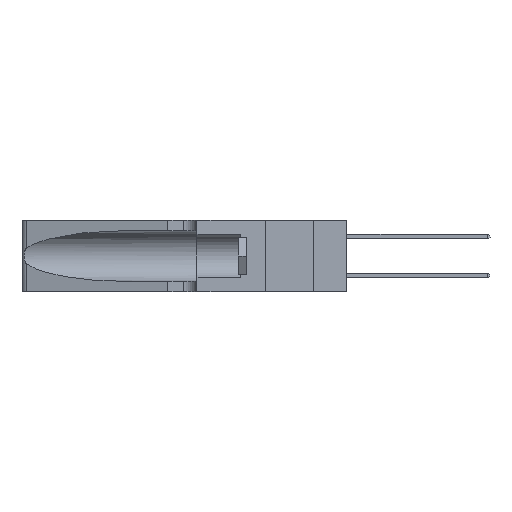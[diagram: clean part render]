
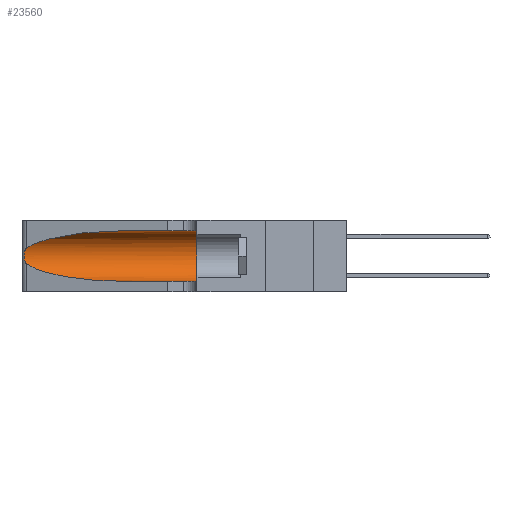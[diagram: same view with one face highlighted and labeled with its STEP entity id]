
A CAD part, left-side view. The second image highlights one B-rep face of the part: STEP entity #23560.
In plain terms, the highlighted cylindrical face has radius 3.308 mm (diameter 6.617 mm), a partial arc.
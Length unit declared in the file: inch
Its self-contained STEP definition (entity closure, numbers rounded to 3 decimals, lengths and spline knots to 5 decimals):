
#1536 = CARTESIAN_POINT ( 'NONE',  ( 0.1305, 0.35, 0.185 ) ) ;
#1537 = ORIENTED_EDGE ( 'NONE', *, *, #2517, .T. ) ;
#1906 = VECTOR ( 'NONE', #22096, 39.37008 ) ;
#1913 =( BOUNDED_CURVE ( )  B_SPLINE_CURVE ( 3, ( #11397, #3986, #19092, #2240 ),
 .UNSPECIFIED., .F., .T. ) 
 B_SPLINE_CURVE_WITH_KNOTS ( ( 4, 4 ),
 ( 1.5708, 2.84003 ),
 .UNSPECIFIED. ) 
 CURVE ( )  GEOMETRIC_REPRESENTATION_ITEM ( )  RATIONAL_B_SPLINE_CURVE ( ( 1., 0.87, 0.87, 1. ) ) 
 REPRESENTATION_ITEM ( '' )  );
#2240 = CARTESIAN_POINT ( 'NONE',  ( 0.25487, 1.22718, 0.22369 ) ) ;
#2402 = CARTESIAN_POINT ( 'NONE',  ( 0.25789, 1.23486, 0.15765 ) ) ;
#2517 = EDGE_CURVE ( 'NONE', #20224, #18466, #10002, .T. ) ;
#2695 = CARTESIAN_POINT ( 'NONE',  ( 0.25487, 1.22718, 0.14631 ) ) ;
#3182 = CARTESIAN_POINT ( 'NONE',  ( 0.25487, 1.22718, 0.14631 ) ) ;
#3450 = DIRECTION ( 'NONE',  ( 0., 1., 0. ) ) ;
#3831 = CIRCLE ( 'NONE', #10021, 0.13025 ) ;
#3986 = CARTESIAN_POINT ( 'NONE',  ( 0.18966, 0.96281, 0.31525 ) ) ;
#4203 = VERTEX_POINT ( 'NONE', #20815 ) ;
#4675 = AXIS2_PLACEMENT_3D ( 'NONE', #20613, #13073, #16848 ) ;
#4845 = VECTOR ( 'NONE', #14578, 39.37008 ) ;
#5646 = B_SPLINE_CURVE_WITH_KNOTS ( 'NONE', 3,
 ( #23398, #12052, #15802, #23474, #6324, #13970, #11973, #15642, #17812, #6080, #2402, #17571, #23313, #7895 ),
 .UNSPECIFIED., .F., .F.,
 ( 4, 2, 2, 2, 2, 2, 4 ),
 ( 0., 0.00027, 0.00053, 0.00107, 0.0016, 0.00187, 0.00214 ),
 .UNSPECIFIED. ) ;
#5675 = EDGE_CURVE ( 'NONE', #18481, #15264, #1913, .T. ) ;
#6080 = CARTESIAN_POINT ( 'NONE',  ( 0.25856, 1.23593, 0.16098 ) ) ;
#6324 = CARTESIAN_POINT ( 'NONE',  ( 0.25854, 1.2359, 0.20912 ) ) ;
#6445 = CARTESIAN_POINT ( 'NONE',  ( 0.1305, 0.35, 0.31525 ) ) ;
#6606 = CARTESIAN_POINT ( 'NONE',  ( 0.1305, 0.72297, 0.05475 ) ) ;
#6783 = CARTESIAN_POINT ( 'NONE',  ( 0.1305, 1.61858, 0.05475 ) ) ;
#6991 = ORIENTED_EDGE ( 'NONE', *, *, #23444, .T. ) ;
#7621 = EDGE_CURVE ( 'NONE', #19948, #4203, #3831, .T. ) ;
#7828 = LINE ( 'NONE', #9065, #4845 ) ;
#7895 = CARTESIAN_POINT ( 'NONE',  ( 0.25487, 1.22718, 0.14631 ) ) ;
#8042 = ORIENTED_EDGE ( 'NONE', *, *, #15702, .T. ) ;
#8195 = CARTESIAN_POINT ( 'NONE',  ( 0.18966, 0.96281, 0.05475 ) ) ;
#9065 = CARTESIAN_POINT ( 'NONE',  ( 0.1305, 1.61858, 0.31525 ) ) ;
#10002 =( BOUNDED_CURVE ( )  B_SPLINE_CURVE ( 3, ( #2695, #21771, #8195, #6606 ),
 .UNSPECIFIED., .F., .F. ) 
 B_SPLINE_CURVE_WITH_KNOTS ( ( 4, 4 ),
 ( 3.44316, 4.71239 ),
 .UNSPECIFIED. ) 
 CURVE ( )  GEOMETRIC_REPRESENTATION_ITEM ( )  RATIONAL_B_SPLINE_CURVE ( ( 1., 0.87, 0.87, 1. ) ) 
 REPRESENTATION_ITEM ( '' )  );
#10021 = AXIS2_PLACEMENT_3D ( 'NONE', #1536, #3450, #16776 ) ;
#11397 = CARTESIAN_POINT ( 'NONE',  ( 0.1305, 0.72297, 0.31525 ) ) ;
#11741 = CARTESIAN_POINT ( 'NONE',  ( 0.1305, 0.72297, 0.31525 ) ) ;
#11766 = ORIENTED_EDGE ( 'NONE', *, *, #24128, .F. ) ;
#11973 = CARTESIAN_POINT ( 'NONE',  ( 0.26075, 1.23896, 0.19203 ) ) ;
#12052 = CARTESIAN_POINT ( 'NONE',  ( 0.25555, 1.22994, 0.2215 ) ) ;
#13073 = DIRECTION ( 'NONE',  ( 0., -1., 0. ) ) ;
#13970 = CARTESIAN_POINT ( 'NONE',  ( 0.26018, 1.23835, 0.19895 ) ) ;
#14418 = CYLINDRICAL_SURFACE ( 'NONE', #4675, 0.13025 ) ;
#14571 = CARTESIAN_POINT ( 'NONE',  ( 0.25487, 1.22718, 0.22369 ) ) ;
#14578 = DIRECTION ( 'NONE',  ( 0., -1., 0. ) ) ;
#15264 = VERTEX_POINT ( 'NONE', #14571 ) ;
#15642 = CARTESIAN_POINT ( 'NONE',  ( 0.26075, 1.23896, 0.178 ) ) ;
#15702 = EDGE_CURVE ( 'NONE', #15264, #20224, #5646, .T. ) ;
#15802 = CARTESIAN_POINT ( 'NONE',  ( 0.25639, 1.23184, 0.21858 ) ) ;
#16776 = DIRECTION ( 'NONE',  ( 0., 0., 1. ) ) ;
#16848 = DIRECTION ( 'NONE',  ( 0., 0., -1. ) ) ;
#17571 = CARTESIAN_POINT ( 'NONE',  ( 0.25639, 1.23186, 0.15144 ) ) ;
#17812 = CARTESIAN_POINT ( 'NONE',  ( 0.26017, 1.23833, 0.17102 ) ) ;
#18466 = VERTEX_POINT ( 'NONE', #23331 ) ;
#18481 = VERTEX_POINT ( 'NONE', #11741 ) ;
#19092 = CARTESIAN_POINT ( 'NONE',  ( 0.2373, 1.15595, 0.28018 ) ) ;
#19531 = FACE_OUTER_BOUND ( 'NONE', #20914, .T. ) ;
#19823 = LINE ( 'NONE', #6783, #1906 ) ;
#19948 = VERTEX_POINT ( 'NONE', #6445 ) ;
#20224 = VERTEX_POINT ( 'NONE', #3182 ) ;
#20613 = CARTESIAN_POINT ( 'NONE',  ( 0.1305, 1.61858, 0.185 ) ) ;
#20815 = CARTESIAN_POINT ( 'NONE',  ( 0.1305, 0.35, 0.05475 ) ) ;
#20914 = EDGE_LOOP ( 'NONE', ( #23085, #8042, #1537, #6991, #21059, #11766 ) ) ;
#21059 = ORIENTED_EDGE ( 'NONE', *, *, #7621, .F. ) ;
#21771 = CARTESIAN_POINT ( 'NONE',  ( 0.2373, 1.15595, 0.08982 ) ) ;
#22096 = DIRECTION ( 'NONE',  ( 0., -1., 0. ) ) ;
#23085 = ORIENTED_EDGE ( 'NONE', *, *, #5675, .T. ) ;
#23313 = CARTESIAN_POINT ( 'NONE',  ( 0.25555, 1.22993, 0.14849 ) ) ;
#23331 = CARTESIAN_POINT ( 'NONE',  ( 0.1305, 0.72297, 0.05475 ) ) ;
#23398 = CARTESIAN_POINT ( 'NONE',  ( 0.25487, 1.22718, 0.22369 ) ) ;
#23444 = EDGE_CURVE ( 'NONE', #18466, #4203, #19823, .T. ) ;
#23474 = CARTESIAN_POINT ( 'NONE',  ( 0.25787, 1.23484, 0.2124 ) ) ;
#23560 = ADVANCED_FACE ( 'NONE', ( #19531 ), #14418, .F. ) ;
#24128 = EDGE_CURVE ( 'NONE', #18481, #19948, #7828, .T. ) ;
